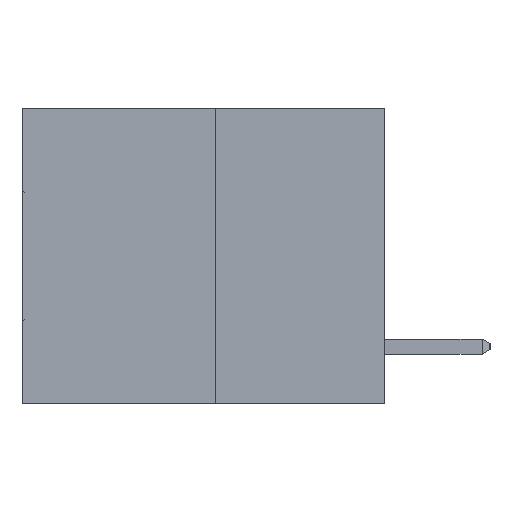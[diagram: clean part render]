
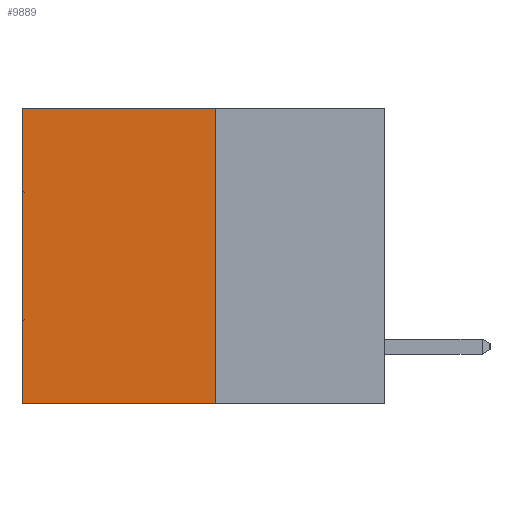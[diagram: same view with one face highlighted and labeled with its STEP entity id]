
A CAD part, left-side view. The second image highlights one B-rep face of the part: STEP entity #9889.
In plain terms, the highlighted planar face has unit normal (-1, 0, 0).
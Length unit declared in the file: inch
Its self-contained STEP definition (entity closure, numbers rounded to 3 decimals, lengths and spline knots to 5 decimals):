
#784 = LINE ( 'NONE', #15723, #2705 ) ;
#1141 = CARTESIAN_POINT ( 'NONE',  ( 0.3165, 0.28, -0.49 ) ) ;
#2705 = VECTOR ( 'NONE', #18204, 39.37008 ) ;
#2727 = DIRECTION ( 'NONE',  ( 0., 1., 0. ) ) ;
#3020 = CARTESIAN_POINT ( 'NONE',  ( 0.3165, 0.6, -0.49 ) ) ;
#4152 = FACE_OUTER_BOUND ( 'NONE', #12998, .T. ) ;
#4574 = CARTESIAN_POINT ( 'NONE',  ( 0.3165, 0.28, 0. ) ) ;
#5905 = DIRECTION ( 'NONE',  ( 0., 0., -1. ) ) ;
#6707 = VERTEX_POINT ( 'NONE', #4574 ) ;
#6743 = EDGE_CURVE ( 'NONE', #9564, #30707, #17320, .T. ) ;
#9244 = DIRECTION ( 'NONE',  ( 0., 1., 0. ) ) ;
#9564 = VERTEX_POINT ( 'NONE', #31648 ) ;
#9889 = ADVANCED_FACE ( 'NONE', ( #4152 ), #20650, .F. ) ;
#10425 = ORIENTED_EDGE ( 'NONE', *, *, #21893, .T. ) ;
#12998 = EDGE_LOOP ( 'NONE', ( #22520, #26562, #22679, #10425 ) ) ;
#13742 = CARTESIAN_POINT ( 'NONE',  ( 0.3165, 0.28, -0.49 ) ) ;
#14968 = AXIS2_PLACEMENT_3D ( 'NONE', #1141, #18500, #5905 ) ;
#15723 = CARTESIAN_POINT ( 'NONE',  ( 0.3165, 0.6, -0.49 ) ) ;
#16543 = DIRECTION ( 'NONE',  ( 0., 0., -1. ) ) ;
#16556 = VECTOR ( 'NONE', #2727, 39.37008 ) ;
#16855 = VECTOR ( 'NONE', #9244, 39.37008 ) ;
#17320 = LINE ( 'NONE', #24700, #16556 ) ;
#17366 = EDGE_CURVE ( 'NONE', #21988, #30707, #784, .T. ) ;
#17437 = CARTESIAN_POINT ( 'NONE',  ( 0.3165, 0.6, 0. ) ) ;
#18204 = DIRECTION ( 'NONE',  ( 0., 0., -1. ) ) ;
#18454 = EDGE_CURVE ( 'NONE', #6707, #9564, #24212, .T. ) ;
#18500 = DIRECTION ( 'NONE',  ( 1., 0., 0. ) ) ;
#20650 = PLANE ( 'NONE',  #14968 ) ;
#21128 = VECTOR ( 'NONE', #16543, 39.37008 ) ;
#21893 = EDGE_CURVE ( 'NONE', #6707, #21988, #28066, .T. ) ;
#21988 = VERTEX_POINT ( 'NONE', #17437 ) ;
#22520 = ORIENTED_EDGE ( 'NONE', *, *, #17366, .T. ) ;
#22679 = ORIENTED_EDGE ( 'NONE', *, *, #18454, .F. ) ;
#24212 = LINE ( 'NONE', #13742, #21128 ) ;
#24700 = CARTESIAN_POINT ( 'NONE',  ( 0.3165, 0.28, -0.49 ) ) ;
#26562 = ORIENTED_EDGE ( 'NONE', *, *, #6743, .F. ) ;
#28066 = LINE ( 'NONE', #31601, #16855 ) ;
#30707 = VERTEX_POINT ( 'NONE', #3020 ) ;
#31601 = CARTESIAN_POINT ( 'NONE',  ( 0.3165, 0.28, 0. ) ) ;
#31648 = CARTESIAN_POINT ( 'NONE',  ( 0.3165, 0.28, -0.49 ) ) ;
